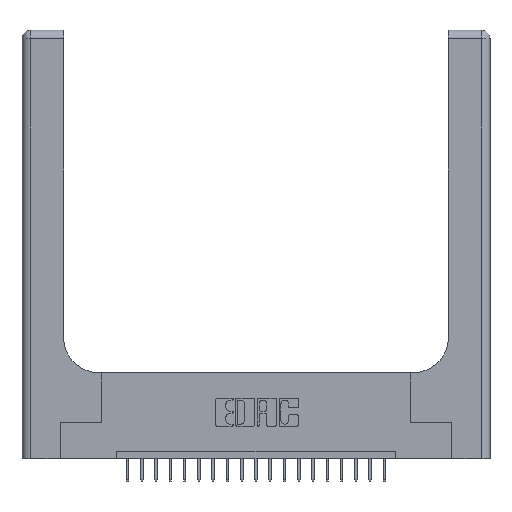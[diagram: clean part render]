
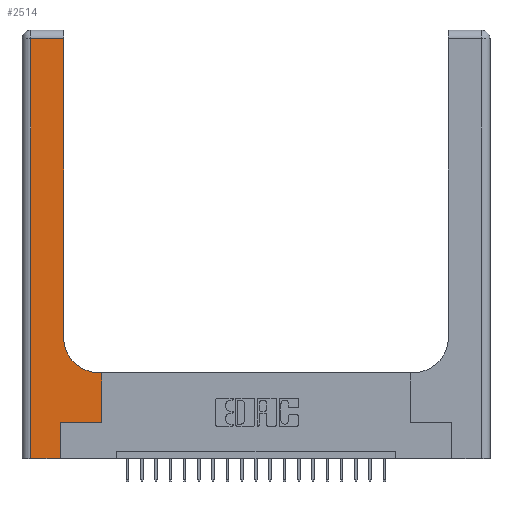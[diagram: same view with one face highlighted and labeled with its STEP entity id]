
A CAD part, top view. The second image highlights one B-rep face of the part: STEP entity #2514.
In plain terms, the highlighted planar face has unit normal (0, 0, 1).
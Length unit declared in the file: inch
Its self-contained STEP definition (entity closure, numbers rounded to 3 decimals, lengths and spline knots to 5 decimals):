
#121 = CARTESIAN_POINT ( 'NONE',  ( 0., 3., 0.37 ) ) ;
#213 = VECTOR ( 'NONE', #15312, 39.37008 ) ;
#446 = DIRECTION ( 'NONE',  ( 0., 1., 0. ) ) ;
#641 = VECTOR ( 'NONE', #12124, 39.37008 ) ;
#747 = DIRECTION ( 'NONE',  ( 0., 0., -1. ) ) ;
#994 = LINE ( 'NONE', #17238, #20696 ) ;
#1294 = DIRECTION ( 'NONE',  ( -1., 0., 0. ) ) ;
#1499 = DIRECTION ( 'NONE',  ( 0., 1., 0. ) ) ;
#1509 = AXIS2_PLACEMENT_3D ( 'NONE', #3086, #22431, #18980 ) ;
#1551 = DIRECTION ( 'NONE',  ( -1., 0., 0. ) ) ;
#1553 = EDGE_CURVE ( 'NONE', #19467, #4335, #8848, .T. ) ;
#2514 = ADVANCED_FACE ( 'NONE', ( #7318 ), #8603, .F. ) ;
#2632 = EDGE_CURVE ( 'NONE', #8798, #20679, #21262, .T. ) ;
#3086 = CARTESIAN_POINT ( 'NONE',  ( 0.5415, 0.85, 0.37 ) ) ;
#3540 = EDGE_CURVE ( 'NONE', #4333, #6732, #994, .T. ) ;
#3660 = AXIS2_PLACEMENT_3D ( 'NONE', #121, #747, #14749 ) ;
#4049 = CARTESIAN_POINT ( 'NONE',  ( 0.269, 0., 0.37 ) ) ;
#4333 = VERTEX_POINT ( 'NONE', #6263 ) ;
#4335 = VERTEX_POINT ( 'NONE', #6581 ) ;
#4493 = LINE ( 'NONE', #10273, #641 ) ;
#5264 = ORIENTED_EDGE ( 'NONE', *, *, #9957, .T. ) ;
#5452 = LINE ( 'NONE', #17367, #20263 ) ;
#5859 = ORIENTED_EDGE ( 'NONE', *, *, #14644, .T. ) ;
#6263 = CARTESIAN_POINT ( 'NONE',  ( 0.2915, 2.94, 0.37 ) ) ;
#6465 = CARTESIAN_POINT ( 'NONE',  ( 0.269, 0.25, 0.37 ) ) ;
#6581 = CARTESIAN_POINT ( 'NONE',  ( 0.5415, 0.6, 0.37 ) ) ;
#6684 = CARTESIAN_POINT ( 'NONE',  ( 0.06, 2.94, 0.37 ) ) ;
#6732 = VERTEX_POINT ( 'NONE', #6684 ) ;
#6946 = VECTOR ( 'NONE', #17145, 39.37008 ) ;
#7318 = FACE_OUTER_BOUND ( 'NONE', #11308, .T. ) ;
#8603 = PLANE ( 'NONE',  #3660 ) ;
#8659 = CARTESIAN_POINT ( 'NONE',  ( 0.2915, 3., 0.37 ) ) ;
#8798 = VERTEX_POINT ( 'NONE', #9382 ) ;
#8848 = LINE ( 'NONE', #18563, #15209 ) ;
#8896 = LINE ( 'NONE', #8659, #11672 ) ;
#9145 = CARTESIAN_POINT ( 'NONE',  ( 0.269, 0., 0.37 ) ) ;
#9335 = CARTESIAN_POINT ( 'NONE',  ( 0.06, 0., 0.37 ) ) ;
#9382 = CARTESIAN_POINT ( 'NONE',  ( 0.269, 0.25, 0.37 ) ) ;
#9734 = ORIENTED_EDGE ( 'NONE', *, *, #3540, .T. ) ;
#9957 = EDGE_CURVE ( 'NONE', #21705, #8798, #18096, .T. ) ;
#10273 = CARTESIAN_POINT ( 'NONE',  ( 0., 0., 0.37 ) ) ;
#11308 = EDGE_LOOP ( 'NONE', ( #21922, #9734, #5859, #14904, #5264, #13671, #13260, #13085, #16478 ) ) ;
#11672 = VECTOR ( 'NONE', #1499, 39.37008 ) ;
#12106 = VERTEX_POINT ( 'NONE', #18767 ) ;
#12124 = DIRECTION ( 'NONE',  ( 1., 0., 0. ) ) ;
#13085 = ORIENTED_EDGE ( 'NONE', *, *, #1553, .T. ) ;
#13260 = ORIENTED_EDGE ( 'NONE', *, *, #17875, .T. ) ;
#13671 = ORIENTED_EDGE ( 'NONE', *, *, #2632, .T. ) ;
#13712 = CARTESIAN_POINT ( 'NONE',  ( 0.5585, 0.6, 0.37 ) ) ;
#14065 = EDGE_CURVE ( 'NONE', #12106, #4333, #8896, .T. ) ;
#14644 = EDGE_CURVE ( 'NONE', #6732, #21642, #20917, .T. ) ;
#14749 = DIRECTION ( 'NONE',  ( -1., 0., 0. ) ) ;
#14904 = ORIENTED_EDGE ( 'NONE', *, *, #15270, .T. ) ;
#15159 = CIRCLE ( 'NONE', #1509, 0.25 ) ;
#15209 = VECTOR ( 'NONE', #1294, 39.37008 ) ;
#15234 = EDGE_CURVE ( 'NONE', #4335, #12106, #15159, .T. ) ;
#15270 = EDGE_CURVE ( 'NONE', #21642, #21705, #4493, .T. ) ;
#15312 = DIRECTION ( 'NONE',  ( 1., 0., 0. ) ) ;
#15397 = DIRECTION ( 'NONE',  ( 0., 1., 0. ) ) ;
#16291 = CARTESIAN_POINT ( 'NONE',  ( 0.06, 3., 0.37 ) ) ;
#16478 = ORIENTED_EDGE ( 'NONE', *, *, #15234, .T. ) ;
#16903 = CARTESIAN_POINT ( 'NONE',  ( 0.5585, 0.25, 0.37 ) ) ;
#17145 = DIRECTION ( 'NONE',  ( 0., -1., 0. ) ) ;
#17238 = CARTESIAN_POINT ( 'NONE',  ( 0., 2.94, 0.37 ) ) ;
#17367 = CARTESIAN_POINT ( 'NONE',  ( 0.5585, 0.25, 0.37 ) ) ;
#17875 = EDGE_CURVE ( 'NONE', #20679, #19467, #5452, .T. ) ;
#18096 = LINE ( 'NONE', #9145, #20579 ) ;
#18563 = CARTESIAN_POINT ( 'NONE',  ( 0.2915, 0.6, 0.37 ) ) ;
#18767 = CARTESIAN_POINT ( 'NONE',  ( 0.2915, 0.85, 0.37 ) ) ;
#18980 = DIRECTION ( 'NONE',  ( 1., 0., 0. ) ) ;
#19467 = VERTEX_POINT ( 'NONE', #13712 ) ;
#20263 = VECTOR ( 'NONE', #15397, 39.37008 ) ;
#20579 = VECTOR ( 'NONE', #446, 39.37008 ) ;
#20679 = VERTEX_POINT ( 'NONE', #16903 ) ;
#20696 = VECTOR ( 'NONE', #1551, 39.37008 ) ;
#20917 = LINE ( 'NONE', #16291, #6946 ) ;
#21262 = LINE ( 'NONE', #6465, #213 ) ;
#21642 = VERTEX_POINT ( 'NONE', #9335 ) ;
#21705 = VERTEX_POINT ( 'NONE', #4049 ) ;
#21922 = ORIENTED_EDGE ( 'NONE', *, *, #14065, .T. ) ;
#22431 = DIRECTION ( 'NONE',  ( 0., 0., -1. ) ) ;
